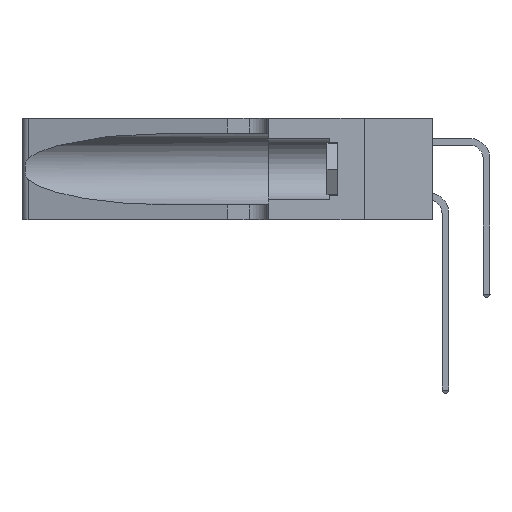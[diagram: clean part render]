
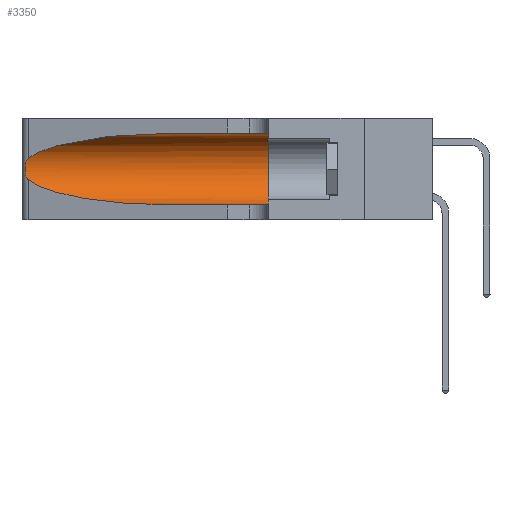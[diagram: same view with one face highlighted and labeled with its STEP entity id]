
A CAD part, left-side view. The second image highlights one B-rep face of the part: STEP entity #3350.
In plain terms, the highlighted cylindrical face has radius 3.308 mm (diameter 6.617 mm), a partial arc.
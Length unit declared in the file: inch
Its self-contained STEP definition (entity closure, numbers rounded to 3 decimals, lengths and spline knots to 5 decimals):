
#370 = CARTESIAN_POINT ( 'NONE',  ( 0.1305, 0.35, 0.185 ) ) ;
#740 =( BOUNDED_CURVE ( )  B_SPLINE_CURVE ( 3, ( #30254, #33640, #13571, #36985 ),
 .UNSPECIFIED., .F., .F. ) 
 B_SPLINE_CURVE_WITH_KNOTS ( ( 4, 4 ),
 ( 1.5708, 2.84003 ),
 .UNSPECIFIED. ) 
 CURVE ( )  GEOMETRIC_REPRESENTATION_ITEM ( )  RATIONAL_B_SPLINE_CURVE ( ( 1., 0.87, 0.87, 1. ) ) 
 REPRESENTATION_ITEM ( '' )  );
#1494 = CARTESIAN_POINT ( 'NONE',  ( 0.25789, 1.23486, 0.15765 ) ) ;
#1539 = CARTESIAN_POINT ( 'NONE',  ( 0.25487, 1.22718, 0.14631 ) ) ;
#2384 = VERTEX_POINT ( 'NONE', #42984 ) ;
#3125 = DIRECTION ( 'NONE',  ( 0., -1., 0. ) ) ;
#3350 = ADVANCED_FACE ( 'NONE', ( #5013 ), #3959, .F. ) ;
#3421 =( BOUNDED_CURVE ( )  B_SPLINE_CURVE ( 3, ( #31098, #4348, #7562, #11049 ),
 .UNSPECIFIED., .F., .F. ) 
 B_SPLINE_CURVE_WITH_KNOTS ( ( 4, 4 ),
 ( 3.44316, 4.71239 ),
 .UNSPECIFIED. ) 
 CURVE ( )  GEOMETRIC_REPRESENTATION_ITEM ( )  RATIONAL_B_SPLINE_CURVE ( ( 1., 0.87, 0.87, 1. ) ) 
 REPRESENTATION_ITEM ( '' )  );
#3745 = DIRECTION ( 'NONE',  ( 0., 0., 1. ) ) ;
#3959 = CYLINDRICAL_SURFACE ( 'NONE', #13233, 0.13025 ) ;
#4348 = CARTESIAN_POINT ( 'NONE',  ( 0.2373, 1.15595, 0.08982 ) ) ;
#4890 = CARTESIAN_POINT ( 'NONE',  ( 0.25555, 1.22993, 0.14849 ) ) ;
#5013 = FACE_OUTER_BOUND ( 'NONE', #24874, .T. ) ;
#5069 = EDGE_CURVE ( 'NONE', #22402, #23266, #3421, .T. ) ;
#5413 = VERTEX_POINT ( 'NONE', #42744 ) ;
#5995 = AXIS2_PLACEMENT_3D ( 'NONE', #370, #23750, #3745 ) ;
#6327 = CARTESIAN_POINT ( 'NONE',  ( 0.1305, 0.72297, 0.05475 ) ) ;
#6523 = CARTESIAN_POINT ( 'NONE',  ( 0.1305, 1.61858, 0.185 ) ) ;
#7542 = CARTESIAN_POINT ( 'NONE',  ( 0.1305, 1.61858, 0.31525 ) ) ;
#7562 = CARTESIAN_POINT ( 'NONE',  ( 0.18966, 0.96281, 0.05475 ) ) ;
#11049 = CARTESIAN_POINT ( 'NONE',  ( 0.1305, 0.72297, 0.05475 ) ) ;
#11443 = CARTESIAN_POINT ( 'NONE',  ( 0.25787, 1.23484, 0.2124 ) ) ;
#12550 = EDGE_CURVE ( 'NONE', #5413, #38194, #740, .T. ) ;
#12659 = CIRCLE ( 'NONE', #5995, 0.13025 ) ;
#12662 = CARTESIAN_POINT ( 'NONE',  ( 0.25487, 1.22718, 0.22369 ) ) ;
#12683 = ORIENTED_EDGE ( 'NONE', *, *, #36920, .T. ) ;
#13061 = B_SPLINE_CURVE_WITH_KNOTS ( 'NONE', 3,
 ( #24752, #24614, #31518, #11443, #34851, #14819, #38221, #18165, #41576, #21535, #1494, #24876, #4890, #28250 ),
 .UNSPECIFIED., .F., .F.,
 ( 4, 2, 2, 2, 2, 2, 4 ),
 ( 0., 0.00027, 0.00053, 0.00107, 0.0016, 0.00187, 0.00214 ),
 .UNSPECIFIED. ) ;
#13233 = AXIS2_PLACEMENT_3D ( 'NONE', #6523, #3125, #36462 ) ;
#13571 = CARTESIAN_POINT ( 'NONE',  ( 0.2373, 1.15595, 0.28018 ) ) ;
#14243 = DIRECTION ( 'NONE',  ( 0., -1., 0. ) ) ;
#14819 = CARTESIAN_POINT ( 'NONE',  ( 0.26018, 1.23835, 0.19895 ) ) ;
#16094 = LINE ( 'NONE', #20366, #32843 ) ;
#17362 = EDGE_CURVE ( 'NONE', #5413, #18912, #43246, .T. ) ;
#17500 = EDGE_CURVE ( 'NONE', #38194, #22402, #13061, .T. ) ;
#18165 = CARTESIAN_POINT ( 'NONE',  ( 0.26075, 1.23896, 0.178 ) ) ;
#18912 = VERTEX_POINT ( 'NONE', #38410 ) ;
#20366 = CARTESIAN_POINT ( 'NONE',  ( 0.1305, 1.61858, 0.05475 ) ) ;
#20441 = ORIENTED_EDGE ( 'NONE', *, *, #28815, .F. ) ;
#21535 = CARTESIAN_POINT ( 'NONE',  ( 0.25856, 1.23593, 0.16098 ) ) ;
#22402 = VERTEX_POINT ( 'NONE', #1539 ) ;
#23266 = VERTEX_POINT ( 'NONE', #6327 ) ;
#23721 = DIRECTION ( 'NONE',  ( 0., -1., 0. ) ) ;
#23750 = DIRECTION ( 'NONE',  ( 0., 1., 0. ) ) ;
#24614 = CARTESIAN_POINT ( 'NONE',  ( 0.25555, 1.22994, 0.2215 ) ) ;
#24752 = CARTESIAN_POINT ( 'NONE',  ( 0.25487, 1.22718, 0.22369 ) ) ;
#24874 = EDGE_LOOP ( 'NONE', ( #25278, #31643, #32521, #12683, #20441, #42088 ) ) ;
#24876 = CARTESIAN_POINT ( 'NONE',  ( 0.25639, 1.23186, 0.15144 ) ) ;
#25278 = ORIENTED_EDGE ( 'NONE', *, *, #12550, .T. ) ;
#28250 = CARTESIAN_POINT ( 'NONE',  ( 0.25487, 1.22718, 0.14631 ) ) ;
#28815 = EDGE_CURVE ( 'NONE', #18912, #2384, #12659, .T. ) ;
#30254 = CARTESIAN_POINT ( 'NONE',  ( 0.1305, 0.72297, 0.31525 ) ) ;
#31098 = CARTESIAN_POINT ( 'NONE',  ( 0.25487, 1.22718, 0.14631 ) ) ;
#31518 = CARTESIAN_POINT ( 'NONE',  ( 0.25639, 1.23184, 0.21858 ) ) ;
#31643 = ORIENTED_EDGE ( 'NONE', *, *, #17500, .T. ) ;
#32521 = ORIENTED_EDGE ( 'NONE', *, *, #5069, .T. ) ;
#32843 = VECTOR ( 'NONE', #23721, 39.37008 ) ;
#33640 = CARTESIAN_POINT ( 'NONE',  ( 0.18966, 0.96281, 0.31525 ) ) ;
#34382 = VECTOR ( 'NONE', #14243, 39.37008 ) ;
#34851 = CARTESIAN_POINT ( 'NONE',  ( 0.25854, 1.2359, 0.20912 ) ) ;
#36462 = DIRECTION ( 'NONE',  ( 0., 0., -1. ) ) ;
#36920 = EDGE_CURVE ( 'NONE', #23266, #2384, #16094, .T. ) ;
#36985 = CARTESIAN_POINT ( 'NONE',  ( 0.25487, 1.22718, 0.22369 ) ) ;
#38194 = VERTEX_POINT ( 'NONE', #12662 ) ;
#38221 = CARTESIAN_POINT ( 'NONE',  ( 0.26075, 1.23896, 0.19203 ) ) ;
#38410 = CARTESIAN_POINT ( 'NONE',  ( 0.1305, 0.35, 0.31525 ) ) ;
#41576 = CARTESIAN_POINT ( 'NONE',  ( 0.26017, 1.23833, 0.17102 ) ) ;
#42088 = ORIENTED_EDGE ( 'NONE', *, *, #17362, .F. ) ;
#42744 = CARTESIAN_POINT ( 'NONE',  ( 0.1305, 0.72297, 0.31525 ) ) ;
#42984 = CARTESIAN_POINT ( 'NONE',  ( 0.1305, 0.35, 0.05475 ) ) ;
#43246 = LINE ( 'NONE', #7542, #34382 ) ;
